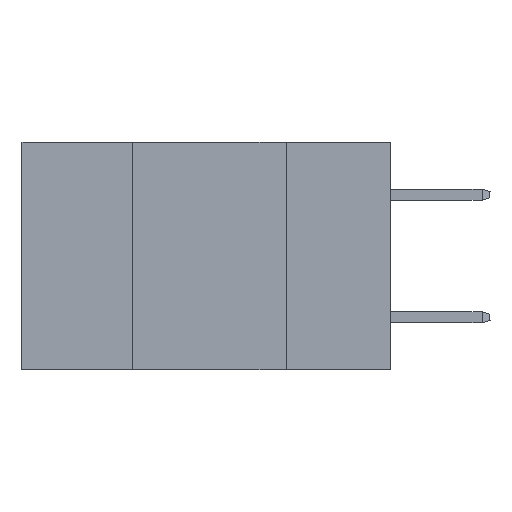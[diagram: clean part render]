
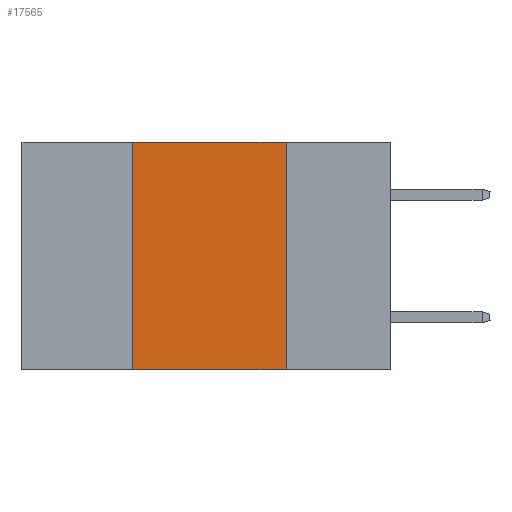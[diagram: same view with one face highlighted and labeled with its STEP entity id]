
A CAD part, left-side view. The second image highlights one B-rep face of the part: STEP entity #17565.
In plain terms, the highlighted planar face has unit normal (-1, 0, 0).
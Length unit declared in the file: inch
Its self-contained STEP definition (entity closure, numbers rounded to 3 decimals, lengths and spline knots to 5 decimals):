
#281 = VECTOR ( 'NONE', #22470, 39.37008 ) ;
#693 = EDGE_CURVE ( 'NONE', #25324, #2875, #20913, .T. ) ;
#953 = CARTESIAN_POINT ( 'NONE',  ( 0., 0.6, 0. ) ) ;
#2875 = VERTEX_POINT ( 'NONE', #22471 ) ;
#3083 = CARTESIAN_POINT ( 'NONE',  ( 0., 0.6, 0. ) ) ;
#4845 = CARTESIAN_POINT ( 'NONE',  ( 0., 0.17, 0. ) ) ;
#6265 = DIRECTION ( 'NONE',  ( 0., 0., 1. ) ) ;
#7260 = PLANE ( 'NONE',  #13562 ) ;
#8378 = ORIENTED_EDGE ( 'NONE', *, *, #15522, .F. ) ;
#9486 = DIRECTION ( 'NONE',  ( 1., 0., 0. ) ) ;
#11897 = EDGE_CURVE ( 'NONE', #2875, #24313, #20436, .T. ) ;
#12723 = EDGE_CURVE ( 'NONE', #25324, #27306, #15189, .T. ) ;
#13299 = CARTESIAN_POINT ( 'NONE',  ( 0., 0.17, 0. ) ) ;
#13562 = AXIS2_PLACEMENT_3D ( 'NONE', #953, #9486, #24166 ) ;
#13597 = CARTESIAN_POINT ( 'NONE',  ( 0., 0.42, -0.37 ) ) ;
#14258 = ORIENTED_EDGE ( 'NONE', *, *, #12723, .T. ) ;
#15189 = LINE ( 'NONE', #26655, #281 ) ;
#15522 = EDGE_CURVE ( 'NONE', #24313, #27306, #19431, .T. ) ;
#16075 = ORIENTED_EDGE ( 'NONE', *, *, #693, .F. ) ;
#16151 = EDGE_LOOP ( 'NONE', ( #8378, #24991, #16075, #14258 ) ) ;
#17565 = ADVANCED_FACE ( 'NONE', ( #19642 ), #7260, .F. ) ;
#18144 = VECTOR ( 'NONE', #19605, 39.37008 ) ;
#18879 = CARTESIAN_POINT ( 'NONE',  ( 0., 0.42, 0. ) ) ;
#19431 = LINE ( 'NONE', #4845, #18144 ) ;
#19605 = DIRECTION ( 'NONE',  ( 0., 0., -1. ) ) ;
#19642 = FACE_OUTER_BOUND ( 'NONE', #16151, .T. ) ;
#20436 = LINE ( 'NONE', #3083, #26744 ) ;
#20893 = DIRECTION ( 'NONE',  ( 0., -1., 0. ) ) ;
#20913 = LINE ( 'NONE', #18879, #21864 ) ;
#21440 = CARTESIAN_POINT ( 'NONE',  ( 0., 0.17, -0.37 ) ) ;
#21864 = VECTOR ( 'NONE', #6265, 39.37008 ) ;
#22470 = DIRECTION ( 'NONE',  ( 0., -1., 0. ) ) ;
#22471 = CARTESIAN_POINT ( 'NONE',  ( 0., 0.42, 0. ) ) ;
#24166 = DIRECTION ( 'NONE',  ( 0., 0., -1. ) ) ;
#24313 = VERTEX_POINT ( 'NONE', #13299 ) ;
#24991 = ORIENTED_EDGE ( 'NONE', *, *, #11897, .F. ) ;
#25324 = VERTEX_POINT ( 'NONE', #13597 ) ;
#26655 = CARTESIAN_POINT ( 'NONE',  ( 0., 0.6, -0.37 ) ) ;
#26744 = VECTOR ( 'NONE', #20893, 39.37008 ) ;
#27306 = VERTEX_POINT ( 'NONE', #21440 ) ;
